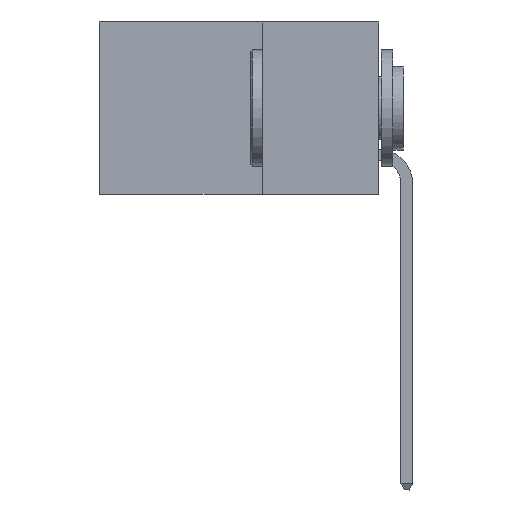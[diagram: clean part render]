
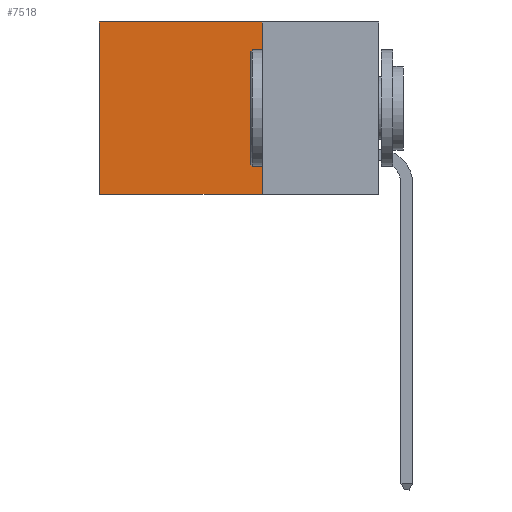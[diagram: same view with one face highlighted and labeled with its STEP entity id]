
A CAD part, left-side view. The second image highlights one B-rep face of the part: STEP entity #7518.
In plain terms, the highlighted planar face has unit normal (-1, 0, 0).
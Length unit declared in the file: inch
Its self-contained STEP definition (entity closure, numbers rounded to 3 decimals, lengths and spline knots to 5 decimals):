
#203 = ORIENTED_EDGE ( 'NONE', *, *, #8878, .F. ) ;
#598 = CARTESIAN_POINT ( 'NONE',  ( 0.2615, 0.25, -0.37 ) ) ;
#645 = CARTESIAN_POINT ( 'NONE',  ( 0.2615, 0.25, 0. ) ) ;
#696 = EDGE_CURVE ( 'NONE', #3073, #8304, #4916, .T. ) ;
#1625 = CARTESIAN_POINT ( 'NONE',  ( 0.2615, 0.6, -0.37 ) ) ;
#1975 = VECTOR ( 'NONE', #4443, 39.37008 ) ;
#2299 = AXIS2_PLACEMENT_3D ( 'NONE', #6997, #3880, #3825 ) ;
#2821 = VERTEX_POINT ( 'NONE', #5917 ) ;
#3073 = VERTEX_POINT ( 'NONE', #645 ) ;
#3136 = DIRECTION ( 'NONE',  ( 0., 0., -1. ) ) ;
#3678 = VECTOR ( 'NONE', #9626, 39.37008 ) ;
#3825 = DIRECTION ( 'NONE',  ( 0., 0., -1. ) ) ;
#3880 = DIRECTION ( 'NONE',  ( 1., 0., 0. ) ) ;
#4053 = LINE ( 'NONE', #1625, #9680 ) ;
#4435 = EDGE_LOOP ( 'NONE', ( #7432, #203, #7680, #5579 ) ) ;
#4443 = DIRECTION ( 'NONE',  ( 0., 0., -1. ) ) ;
#4916 = LINE ( 'NONE', #6354, #3678 ) ;
#5203 = CARTESIAN_POINT ( 'NONE',  ( 0.2615, 0.6, -0.37 ) ) ;
#5290 = LINE ( 'NONE', #598, #1975 ) ;
#5579 = ORIENTED_EDGE ( 'NONE', *, *, #696, .T. ) ;
#5917 = CARTESIAN_POINT ( 'NONE',  ( 0.2615, 0.25, -0.37 ) ) ;
#6214 = CARTESIAN_POINT ( 'NONE',  ( 0.2615, 0.6, 0. ) ) ;
#6354 = CARTESIAN_POINT ( 'NONE',  ( 0.2615, 0.25, 0. ) ) ;
#6451 = VECTOR ( 'NONE', #9236, 39.37008 ) ;
#6997 = CARTESIAN_POINT ( 'NONE',  ( 0.2615, 0.25, -0.37 ) ) ;
#7046 = FACE_OUTER_BOUND ( 'NONE', #4435, .T. ) ;
#7147 = VERTEX_POINT ( 'NONE', #5203 ) ;
#7432 = ORIENTED_EDGE ( 'NONE', *, *, #10484, .T. ) ;
#7518 = ADVANCED_FACE ( 'NONE', ( #7046 ), #10202, .F. ) ;
#7680 = ORIENTED_EDGE ( 'NONE', *, *, #9330, .F. ) ;
#8304 = VERTEX_POINT ( 'NONE', #6214 ) ;
#8878 = EDGE_CURVE ( 'NONE', #2821, #7147, #9298, .T. ) ;
#9236 = DIRECTION ( 'NONE',  ( 0., 1., 0. ) ) ;
#9298 = LINE ( 'NONE', #10058, #6451 ) ;
#9330 = EDGE_CURVE ( 'NONE', #3073, #2821, #5290, .T. ) ;
#9626 = DIRECTION ( 'NONE',  ( 0., 1., 0. ) ) ;
#9680 = VECTOR ( 'NONE', #3136, 39.37008 ) ;
#10058 = CARTESIAN_POINT ( 'NONE',  ( 0.2615, 0.25, -0.37 ) ) ;
#10202 = PLANE ( 'NONE',  #2299 ) ;
#10484 = EDGE_CURVE ( 'NONE', #8304, #7147, #4053, .T. ) ;
